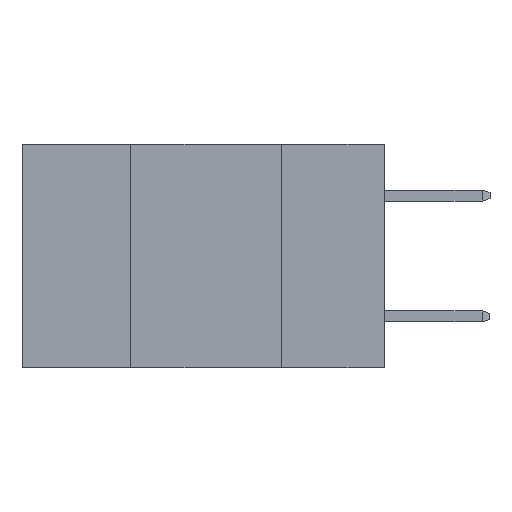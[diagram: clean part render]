
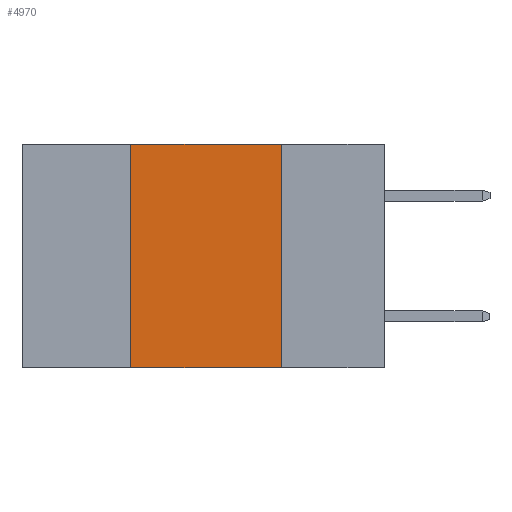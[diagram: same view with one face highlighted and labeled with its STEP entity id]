
A CAD part, left-side view. The second image highlights one B-rep face of the part: STEP entity #4970.
In plain terms, the highlighted planar face has unit normal (-1, 0, 0).
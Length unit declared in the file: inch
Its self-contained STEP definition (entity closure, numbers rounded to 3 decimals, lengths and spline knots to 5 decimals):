
#369 = VERTEX_POINT ( 'NONE', #1020 ) ;
#388 = ORIENTED_EDGE ( 'NONE', *, *, #5434, .T. ) ;
#722 = VECTOR ( 'NONE', #11760, 39.37008 ) ;
#1020 = CARTESIAN_POINT ( 'NONE',  ( 0., 0.17, 0. ) ) ;
#2198 = DIRECTION ( 'NONE',  ( 0., -1., 0. ) ) ;
#2320 = CARTESIAN_POINT ( 'NONE',  ( 0., 0.6, -0.37 ) ) ;
#2609 = ORIENTED_EDGE ( 'NONE', *, *, #10264, .F. ) ;
#3512 = LINE ( 'NONE', #7060, #14368 ) ;
#4231 = EDGE_LOOP ( 'NONE', ( #6303, #10417, #2609, #388 ) ) ;
#4970 = ADVANCED_FACE ( 'NONE', ( #11782 ), #6718, .F. ) ;
#5019 = CARTESIAN_POINT ( 'NONE',  ( 0., 0.42, 0. ) ) ;
#5404 = DIRECTION ( 'NONE',  ( 0., 0., -1. ) ) ;
#5430 = DIRECTION ( 'NONE',  ( 1., 0., 0. ) ) ;
#5434 = EDGE_CURVE ( 'NONE', #7361, #8014, #6361, .T. ) ;
#5929 = DIRECTION ( 'NONE',  ( 0., 0., -1. ) ) ;
#6256 = VECTOR ( 'NONE', #8158, 39.37008 ) ;
#6303 = ORIENTED_EDGE ( 'NONE', *, *, #12083, .F. ) ;
#6361 = LINE ( 'NONE', #2320, #11274 ) ;
#6599 = LINE ( 'NONE', #11452, #6256 ) ;
#6664 = CARTESIAN_POINT ( 'NONE',  ( 0., 0.6, 0. ) ) ;
#6718 = PLANE ( 'NONE',  #14520 ) ;
#7060 = CARTESIAN_POINT ( 'NONE',  ( 0., 0.17, 0. ) ) ;
#7361 = VERTEX_POINT ( 'NONE', #12451 ) ;
#8014 = VERTEX_POINT ( 'NONE', #11341 ) ;
#8158 = DIRECTION ( 'NONE',  ( 0., -1., 0. ) ) ;
#9989 = LINE ( 'NONE', #5019, #722 ) ;
#10264 = EDGE_CURVE ( 'NONE', #7361, #11614, #9989, .T. ) ;
#10417 = ORIENTED_EDGE ( 'NONE', *, *, #10771, .F. ) ;
#10771 = EDGE_CURVE ( 'NONE', #11614, #369, #6599, .T. ) ;
#11274 = VECTOR ( 'NONE', #2198, 39.37008 ) ;
#11341 = CARTESIAN_POINT ( 'NONE',  ( 0., 0.17, -0.37 ) ) ;
#11452 = CARTESIAN_POINT ( 'NONE',  ( 0., 0.6, 0. ) ) ;
#11614 = VERTEX_POINT ( 'NONE', #14007 ) ;
#11760 = DIRECTION ( 'NONE',  ( 0., 0., 1. ) ) ;
#11782 = FACE_OUTER_BOUND ( 'NONE', #4231, .T. ) ;
#12083 = EDGE_CURVE ( 'NONE', #369, #8014, #3512, .T. ) ;
#12451 = CARTESIAN_POINT ( 'NONE',  ( 0., 0.42, -0.37 ) ) ;
#14007 = CARTESIAN_POINT ( 'NONE',  ( 0., 0.42, 0. ) ) ;
#14368 = VECTOR ( 'NONE', #5929, 39.37008 ) ;
#14520 = AXIS2_PLACEMENT_3D ( 'NONE', #6664, #5430, #5404 ) ;
